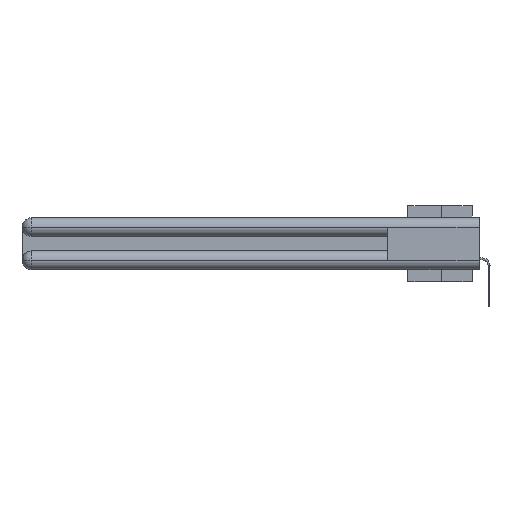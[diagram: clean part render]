
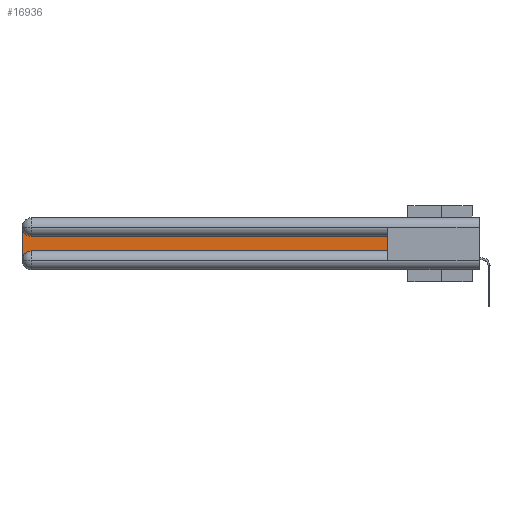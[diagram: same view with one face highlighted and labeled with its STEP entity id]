
A CAD part, left-side view. The second image highlights one B-rep face of the part: STEP entity #16936.
In plain terms, the highlighted planar face has unit normal (-1, 0, 0).
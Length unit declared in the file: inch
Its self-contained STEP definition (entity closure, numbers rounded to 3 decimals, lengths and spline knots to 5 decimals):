
#846 = AXIS2_PLACEMENT_3D ( 'NONE', #9687, #20367, #17147 ) ;
#1491 = VERTEX_POINT ( 'NONE', #9942 ) ;
#2030 = FACE_OUTER_BOUND ( 'NONE', #28534, .T. ) ;
#5177 = AXIS2_PLACEMENT_3D ( 'NONE', #17330, #30613, #28047 ) ;
#6639 = VERTEX_POINT ( 'NONE', #29710 ) ;
#6656 = CARTESIAN_POINT ( 'NONE',  ( 0.075, 2.94, -0.2175 ) ) ;
#7024 = CARTESIAN_POINT ( 'NONE',  ( 0.075, 3., -0.2175 ) ) ;
#7559 = AXIS2_PLACEMENT_3D ( 'NONE', #30330, #18057, #25550 ) ;
#8336 = CARTESIAN_POINT ( 'NONE',  ( 0.075, 0.6, -0.1225 ) ) ;
#8927 = EDGE_CURVE ( 'NONE', #1491, #29332, #22307, .T. ) ;
#9146 = DIRECTION ( 'NONE',  ( 0., 0., 1. ) ) ;
#9433 = CARTESIAN_POINT ( 'NONE',  ( 0.075, 3., -0.2775 ) ) ;
#9596 = EDGE_CURVE ( 'NONE', #6639, #13223, #31941, .T. ) ;
#9687 = CARTESIAN_POINT ( 'NONE',  ( 0.075, 3., -0.1225 ) ) ;
#9726 = CIRCLE ( 'NONE', #7559, 0.06 ) ;
#9942 = CARTESIAN_POINT ( 'NONE',  ( 0.075, 3., -0.0625 ) ) ;
#11370 = VECTOR ( 'NONE', #21840, 39.37008 ) ;
#13223 = VERTEX_POINT ( 'NONE', #29312 ) ;
#13862 = CARTESIAN_POINT ( 'NONE',  ( 0.075, 0.6, -0.2175 ) ) ;
#14190 = LINE ( 'NONE', #13862, #11370 ) ;
#14393 = CARTESIAN_POINT ( 'NONE',  ( 0.075, 0.6, -0.2175 ) ) ;
#15027 = VERTEX_POINT ( 'NONE', #6656 ) ;
#16084 = ORIENTED_EDGE ( 'NONE', *, *, #28128, .T. ) ;
#16451 = LINE ( 'NONE', #14393, #17362 ) ;
#16936 = ADVANCED_FACE ( 'NONE', ( #2030 ), #30421, .F. ) ;
#17067 = ORIENTED_EDGE ( 'NONE', *, *, #32418, .T. ) ;
#17147 = DIRECTION ( 'NONE',  ( 0., 0., -1. ) ) ;
#17330 = CARTESIAN_POINT ( 'NONE',  ( 0.075, 2.94, -0.2775 ) ) ;
#17362 = VECTOR ( 'NONE', #9146, 39.37008 ) ;
#17385 = VECTOR ( 'NONE', #26662, 39.37008 ) ;
#18057 = DIRECTION ( 'NONE',  ( 1., 0., 0. ) ) ;
#18521 = CARTESIAN_POINT ( 'NONE',  ( 0.075, 0.6, -0.2175 ) ) ;
#20253 = DIRECTION ( 'NONE',  ( 0., 0., -1. ) ) ;
#20367 = DIRECTION ( 'NONE',  ( 1., 0., 0. ) ) ;
#20723 = ORIENTED_EDGE ( 'NONE', *, *, #9596, .T. ) ;
#21840 = DIRECTION ( 'NONE',  ( 0., -1., 0. ) ) ;
#21921 = ORIENTED_EDGE ( 'NONE', *, *, #22341, .T. ) ;
#22307 = LINE ( 'NONE', #7024, #26031 ) ;
#22341 = EDGE_CURVE ( 'NONE', #13223, #1491, #9726, .T. ) ;
#23381 = EDGE_CURVE ( 'NONE', #30171, #6639, #16451, .T. ) ;
#25550 = DIRECTION ( 'NONE',  ( 0., 0., -1. ) ) ;
#26031 = VECTOR ( 'NONE', #20253, 39.37008 ) ;
#26662 = DIRECTION ( 'NONE',  ( 0., 1., 0. ) ) ;
#26876 = CIRCLE ( 'NONE', #5177, 0.06 ) ;
#28047 = DIRECTION ( 'NONE',  ( 0., 0., -1. ) ) ;
#28128 = EDGE_CURVE ( 'NONE', #29332, #15027, #26876, .T. ) ;
#28534 = EDGE_LOOP ( 'NONE', ( #20723, #21921, #32722, #16084, #17067, #30605 ) ) ;
#29312 = CARTESIAN_POINT ( 'NONE',  ( 0.075, 2.94, -0.1225 ) ) ;
#29332 = VERTEX_POINT ( 'NONE', #9433 ) ;
#29710 = CARTESIAN_POINT ( 'NONE',  ( 0.075, 0.6, -0.1225 ) ) ;
#30171 = VERTEX_POINT ( 'NONE', #18521 ) ;
#30330 = CARTESIAN_POINT ( 'NONE',  ( 0.075, 2.94, -0.0625 ) ) ;
#30421 = PLANE ( 'NONE',  #846 ) ;
#30605 = ORIENTED_EDGE ( 'NONE', *, *, #23381, .T. ) ;
#30613 = DIRECTION ( 'NONE',  ( 1., 0., 0. ) ) ;
#31941 = LINE ( 'NONE', #8336, #17385 ) ;
#32418 = EDGE_CURVE ( 'NONE', #15027, #30171, #14190, .T. ) ;
#32722 = ORIENTED_EDGE ( 'NONE', *, *, #8927, .T. ) ;
